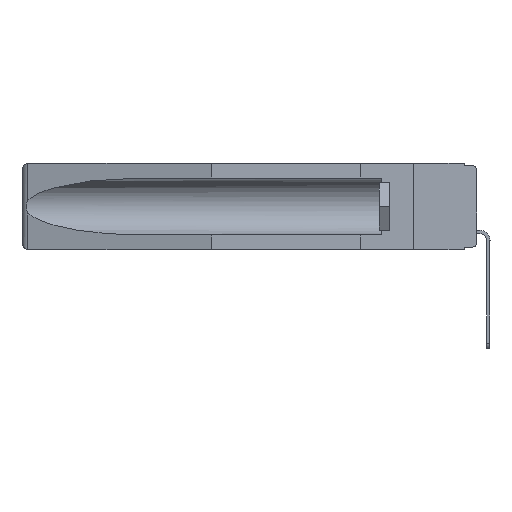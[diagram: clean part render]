
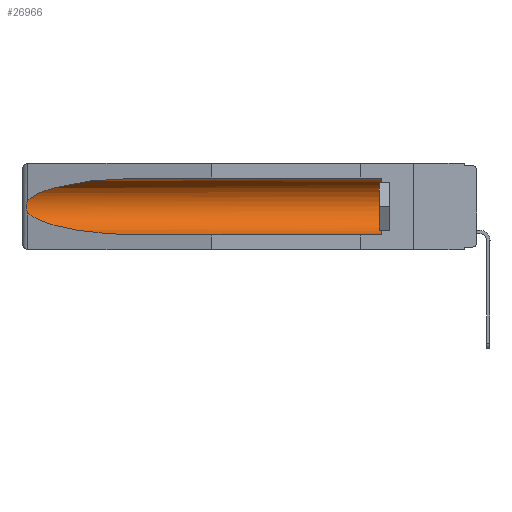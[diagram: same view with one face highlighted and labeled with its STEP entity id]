
A CAD part, left-side view. The second image highlights one B-rep face of the part: STEP entity #26966.
In plain terms, the highlighted cylindrical face has radius 2.857 mm (diameter 5.715 mm), a partial arc.
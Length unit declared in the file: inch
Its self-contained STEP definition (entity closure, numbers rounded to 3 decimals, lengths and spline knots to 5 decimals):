
#181 = CARTESIAN_POINT ( 'NONE',  ( 0.155, -0.30754, -0.059 ) ) ;
#844 = ORIENTED_EDGE ( 'NONE', *, *, #2959, .T. ) ;
#1197 = CARTESIAN_POINT ( 'NONE',  ( 0.25451, 1.48313, -0.24835 ) ) ;
#1287 = ORIENTED_EDGE ( 'NONE', *, *, #22114, .T. ) ;
#1348 =( BOUNDED_CURVE ( )  B_SPLINE_CURVE ( 3, ( #23213, #11616, #13878, #18756 ),
 .UNSPECIFIED., .F., .T. ) 
 B_SPLINE_CURVE_WITH_KNOTS ( ( 4, 4 ),
 ( 4.71239, 6.08839 ),
 .UNSPECIFIED. ) 
 CURVE ( )  GEOMETRIC_REPRESENTATION_ITEM ( )  RATIONAL_B_SPLINE_CURVE ( ( 1., 0.848, 0.848, 1. ) ) 
 REPRESENTATION_ITEM ( '' )  );
#1654 = CARTESIAN_POINT ( 'NONE',  ( 0.155, -0.30754, -0.284 ) ) ;
#1727 = DIRECTION ( 'NONE',  ( 0., 1., 0. ) ) ;
#1789 = DIRECTION ( 'NONE',  ( 0., 1., 0. ) ) ;
#1942 = VERTEX_POINT ( 'NONE', #18620 ) ;
#2274 = CARTESIAN_POINT ( 'NONE',  ( 0.26537, 1.52718, -0.14972 ) ) ;
#2559 = AXIS2_PLACEMENT_3D ( 'NONE', #14769, #1727, #10505 ) ;
#2594 = CARTESIAN_POINT ( 'NONE',  ( 0.155, 1.07973, -0.059 ) ) ;
#2728 = CARTESIAN_POINT ( 'NONE',  ( 0.26537, 1.52718, -0.19328 ) ) ;
#2849 = VECTOR ( 'NONE', #1789, 39.37008 ) ;
#2959 = EDGE_CURVE ( 'NONE', #11319, #1942, #20150, .T. ) ;
#3014 = CARTESIAN_POINT ( 'NONE',  ( 0.26537, 1.52718, -0.14972 ) ) ;
#5617 = CARTESIAN_POINT ( 'NONE',  ( 0.155, 0.126, -0.059 ) ) ;
#6035 = CYLINDRICAL_SURFACE ( 'NONE', #2559, 0.1125 ) ;
#6440 = ORIENTED_EDGE ( 'NONE', *, *, #7394, .T. ) ;
#7394 = EDGE_CURVE ( 'NONE', #14783, #22424, #10183, .T. ) ;
#7954 = CARTESIAN_POINT ( 'NONE',  ( 0.21114, 1.30732, -0.284 ) ) ;
#9786 = CARTESIAN_POINT ( 'NONE',  ( 0.26654, 1.53092, -0.15636 ) ) ;
#9972 = CARTESIAN_POINT ( 'NONE',  ( 0.155, 1.07973, -0.284 ) ) ;
#10183 = CIRCLE ( 'NONE', #27088, 0.1125 ) ;
#10281 = LINE ( 'NONE', #1654, #2849 ) ;
#10505 = DIRECTION ( 'NONE',  ( 0., 0., 1. ) ) ;
#11319 = VERTEX_POINT ( 'NONE', #2274 ) ;
#11616 = CARTESIAN_POINT ( 'NONE',  ( 0.21114, 1.30732, -0.059 ) ) ;
#12007 = CARTESIAN_POINT ( 'NONE',  ( 0.155, 0.126, -0.284 ) ) ;
#12097 = CARTESIAN_POINT ( 'NONE',  ( 0.26537, 1.52718, -0.19328 ) ) ;
#12509 = EDGE_CURVE ( 'NONE', #1942, #15641, #16159, .T. ) ;
#13137 = ORIENTED_EDGE ( 'NONE', *, *, #15594, .T. ) ;
#13614 = CARTESIAN_POINT ( 'NONE',  ( 0.2675, 1.53308, -0.17534 ) ) ;
#13754 = CARTESIAN_POINT ( 'NONE',  ( 0.26655, 1.53094, -0.18657 ) ) ;
#13761 = EDGE_LOOP ( 'NONE', ( #13137, #844, #22205, #26230, #6440, #1287 ) ) ;
#13878 = CARTESIAN_POINT ( 'NONE',  ( 0.25451, 1.48313, -0.09465 ) ) ;
#14037 = CARTESIAN_POINT ( 'NONE',  ( 0.2673, 1.53269, -0.17917 ) ) ;
#14769 = CARTESIAN_POINT ( 'NONE',  ( 0.155, -0.30754, -0.1715 ) ) ;
#14783 = VERTEX_POINT ( 'NONE', #12007 ) ;
#14898 = EDGE_CURVE ( 'NONE', #14783, #15641, #10281, .T. ) ;
#15594 = EDGE_CURVE ( 'NONE', #18330, #11319, #1348, .T. ) ;
#15641 = VERTEX_POINT ( 'NONE', #20771 ) ;
#16159 =( BOUNDED_CURVE ( )  B_SPLINE_CURVE ( 3, ( #12097, #1197, #7954, #9972 ),
 .UNSPECIFIED., .F., .T. ) 
 B_SPLINE_CURVE_WITH_KNOTS ( ( 4, 4 ),
 ( 0.1948, 1.5708 ),
 .UNSPECIFIED. ) 
 CURVE ( )  GEOMETRIC_REPRESENTATION_ITEM ( )  RATIONAL_B_SPLINE_CURVE ( ( 1., 0.848, 0.848, 1. ) ) 
 REPRESENTATION_ITEM ( '' )  );
#18330 = VERTEX_POINT ( 'NONE', #2594 ) ;
#18620 = CARTESIAN_POINT ( 'NONE',  ( 0.26537, 1.52718, -0.19328 ) ) ;
#18756 = CARTESIAN_POINT ( 'NONE',  ( 0.26537, 1.52718, -0.14972 ) ) ;
#19818 = LINE ( 'NONE', #181, #26426 ) ;
#20150 = B_SPLINE_CURVE_WITH_KNOTS ( 'NONE', 3,
 ( #3014, #27082, #9786, #24934, #24797, #13614, #14037, #13754, #22378, #2728 ),
 .UNSPECIFIED., .F., .F.,
 ( 4, 2, 2, 2, 4 ),
 ( 0., 0.00029, 0.00058, 0.00087, 0.00117 ),
 .UNSPECIFIED. ) ;
#20771 = CARTESIAN_POINT ( 'NONE',  ( 0.155, 1.07973, -0.284 ) ) ;
#21261 = CARTESIAN_POINT ( 'NONE',  ( 0.155, 0.126, -0.1715 ) ) ;
#21779 = FACE_OUTER_BOUND ( 'NONE', #13761, .T. ) ;
#22114 = EDGE_CURVE ( 'NONE', #22424, #18330, #19818, .T. ) ;
#22205 = ORIENTED_EDGE ( 'NONE', *, *, #12509, .T. ) ;
#22378 = CARTESIAN_POINT ( 'NONE',  ( 0.26597, 1.5296, -0.19026 ) ) ;
#22424 = VERTEX_POINT ( 'NONE', #5617 ) ;
#23143 = DIRECTION ( 'NONE',  ( 0., 0., 1. ) ) ;
#23213 = CARTESIAN_POINT ( 'NONE',  ( 0.155, 1.07973, -0.059 ) ) ;
#24797 = CARTESIAN_POINT ( 'NONE',  ( 0.2675, 1.53308, -0.16763 ) ) ;
#24934 = CARTESIAN_POINT ( 'NONE',  ( 0.2673, 1.5327, -0.16383 ) ) ;
#25273 = DIRECTION ( 'NONE',  ( 0., -1., 0. ) ) ;
#26106 = DIRECTION ( 'NONE',  ( 0., 1., 0. ) ) ;
#26230 = ORIENTED_EDGE ( 'NONE', *, *, #14898, .F. ) ;
#26426 = VECTOR ( 'NONE', #26106, 39.37008 ) ;
#26966 = ADVANCED_FACE ( 'NONE', ( #21779 ), #6035, .F. ) ;
#27082 = CARTESIAN_POINT ( 'NONE',  ( 0.26597, 1.52961, -0.15275 ) ) ;
#27088 = AXIS2_PLACEMENT_3D ( 'NONE', #21261, #25273, #23143 ) ;
